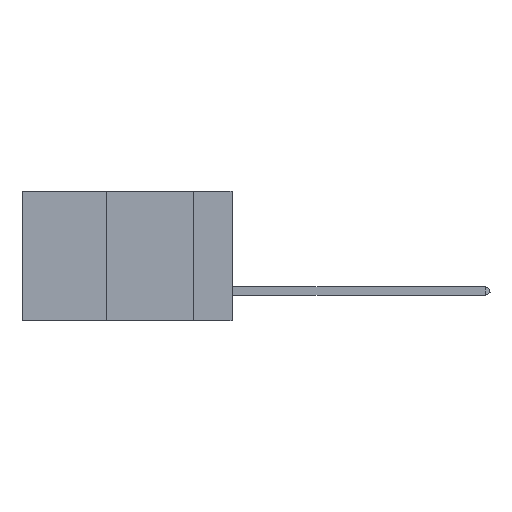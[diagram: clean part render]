
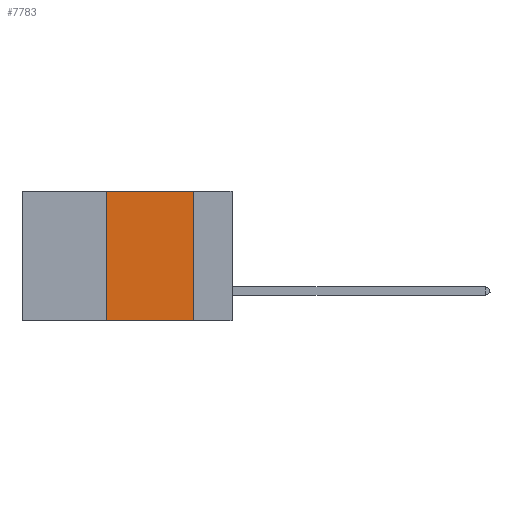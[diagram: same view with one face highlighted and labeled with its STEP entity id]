
A CAD part, left-side view. The second image highlights one B-rep face of the part: STEP entity #7783.
In plain terms, the highlighted planar face has unit normal (-1, 0, 0).
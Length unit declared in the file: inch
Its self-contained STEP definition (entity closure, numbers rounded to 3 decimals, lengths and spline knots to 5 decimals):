
#52 = CARTESIAN_POINT ( 'NONE',  ( 0., 0.36, -0.37 ) ) ;
#107 = DIRECTION ( 'NONE',  ( 0., -1., 0. ) ) ;
#369 = ORIENTED_EDGE ( 'NONE', *, *, #3360, .F. ) ;
#504 = VERTEX_POINT ( 'NONE', #6077 ) ;
#702 = LINE ( 'NONE', #2451, #9332 ) ;
#801 = AXIS2_PLACEMENT_3D ( 'NONE', #10049, #11080, #16094 ) ;
#1708 = CARTESIAN_POINT ( 'NONE',  ( 0., 0.11, 0. ) ) ;
#2451 = CARTESIAN_POINT ( 'NONE',  ( 0., 0.11, 0. ) ) ;
#3360 = EDGE_CURVE ( 'NONE', #8434, #8630, #9791, .T. ) ;
#3656 = PLANE ( 'NONE',  #801 ) ;
#4928 = DIRECTION ( 'NONE',  ( 0., 0., -1. ) ) ;
#5890 = VECTOR ( 'NONE', #12487, 39.37008 ) ;
#6077 = CARTESIAN_POINT ( 'NONE',  ( 0., 0.11, -0.37 ) ) ;
#6651 = ORIENTED_EDGE ( 'NONE', *, *, #13284, .F. ) ;
#6818 = CARTESIAN_POINT ( 'NONE',  ( 0., 0.36, 0. ) ) ;
#7115 = FACE_OUTER_BOUND ( 'NONE', #8035, .T. ) ;
#7783 = ADVANCED_FACE ( 'NONE', ( #7115 ), #3656, .F. ) ;
#8035 = EDGE_LOOP ( 'NONE', ( #6651, #12615, #369, #16070 ) ) ;
#8230 = EDGE_CURVE ( 'NONE', #8434, #504, #10790, .T. ) ;
#8434 = VERTEX_POINT ( 'NONE', #52 ) ;
#8630 = VERTEX_POINT ( 'NONE', #6818 ) ;
#9332 = VECTOR ( 'NONE', #4928, 39.37008 ) ;
#9791 = LINE ( 'NONE', #15078, #5890 ) ;
#10049 = CARTESIAN_POINT ( 'NONE',  ( 0., 0.6, 0. ) ) ;
#10434 = DIRECTION ( 'NONE',  ( 0., -1., 0. ) ) ;
#10670 = VECTOR ( 'NONE', #10434, 39.37008 ) ;
#10790 = LINE ( 'NONE', #11297, #15340 ) ;
#11080 = DIRECTION ( 'NONE',  ( 1., 0., 0. ) ) ;
#11297 = CARTESIAN_POINT ( 'NONE',  ( 0., 0.6, -0.37 ) ) ;
#12487 = DIRECTION ( 'NONE',  ( 0., 0., 1. ) ) ;
#12615 = ORIENTED_EDGE ( 'NONE', *, *, #14302, .F. ) ;
#12938 = CARTESIAN_POINT ( 'NONE',  ( 0., 0.6, 0. ) ) ;
#13284 = EDGE_CURVE ( 'NONE', #14914, #504, #702, .T. ) ;
#14193 = LINE ( 'NONE', #12938, #10670 ) ;
#14302 = EDGE_CURVE ( 'NONE', #8630, #14914, #14193, .T. ) ;
#14914 = VERTEX_POINT ( 'NONE', #1708 ) ;
#15078 = CARTESIAN_POINT ( 'NONE',  ( 0., 0.36, 0. ) ) ;
#15340 = VECTOR ( 'NONE', #107, 39.37008 ) ;
#16070 = ORIENTED_EDGE ( 'NONE', *, *, #8230, .T. ) ;
#16094 = DIRECTION ( 'NONE',  ( 0., 0., -1. ) ) ;
